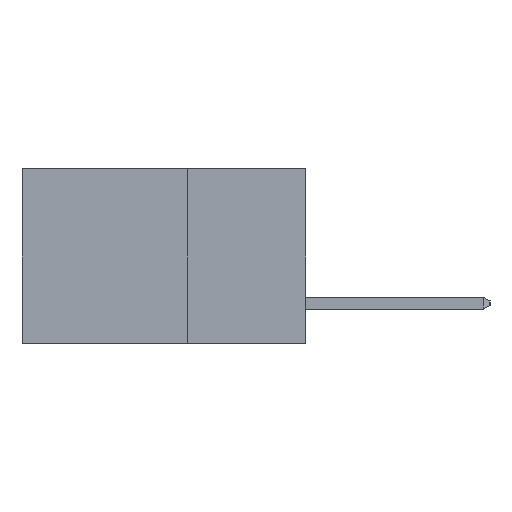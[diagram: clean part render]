
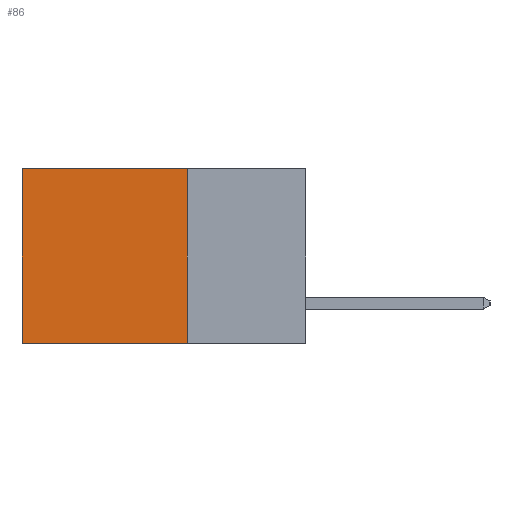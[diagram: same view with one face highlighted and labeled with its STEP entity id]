
A CAD part, left-side view. The second image highlights one B-rep face of the part: STEP entity #86.
In plain terms, the highlighted planar face has unit normal (-1, 0, 0).
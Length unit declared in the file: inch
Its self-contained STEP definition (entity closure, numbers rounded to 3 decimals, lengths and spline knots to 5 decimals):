
#24 = CARTESIAN_POINT ( 'NONE',  ( 0.2615, 0.25, -0.37 ) ) ;
#86 = ADVANCED_FACE ( 'NONE', ( #5015 ), #9644, .F. ) ;
#387 = CARTESIAN_POINT ( 'NONE',  ( 0.2615, 0.6, -0.37 ) ) ;
#1354 = DIRECTION ( 'NONE',  ( 0., 0., -1. ) ) ;
#1418 = AXIS2_PLACEMENT_3D ( 'NONE', #1578, #8172, #13003 ) ;
#1578 = CARTESIAN_POINT ( 'NONE',  ( 0.2615, 0.25, -0.37 ) ) ;
#2103 = EDGE_LOOP ( 'NONE', ( #4500, #5108, #12164, #8286 ) ) ;
#2274 = LINE ( 'NONE', #387, #12182 ) ;
#3090 = EDGE_CURVE ( 'NONE', #9852, #3947, #7965, .T. ) ;
#3339 = EDGE_CURVE ( 'NONE', #11125, #7864, #6919, .T. ) ;
#3477 = VECTOR ( 'NONE', #1354, 39.37008 ) ;
#3947 = VERTEX_POINT ( 'NONE', #9550 ) ;
#4035 = VECTOR ( 'NONE', #11109, 39.37008 ) ;
#4500 = ORIENTED_EDGE ( 'NONE', *, *, #14766, .T. ) ;
#4514 = CARTESIAN_POINT ( 'NONE',  ( 0.2615, 0.25, -0.37 ) ) ;
#5015 = FACE_OUTER_BOUND ( 'NONE', #2103, .T. ) ;
#5108 = ORIENTED_EDGE ( 'NONE', *, *, #3339, .F. ) ;
#5744 = DIRECTION ( 'NONE',  ( 0., 1., 0. ) ) ;
#6919 = LINE ( 'NONE', #10249, #9940 ) ;
#7864 = VERTEX_POINT ( 'NONE', #8886 ) ;
#7965 = LINE ( 'NONE', #10849, #4035 ) ;
#8172 = DIRECTION ( 'NONE',  ( 1., 0., 0. ) ) ;
#8286 = ORIENTED_EDGE ( 'NONE', *, *, #3090, .T. ) ;
#8290 = DIRECTION ( 'NONE',  ( 0., 0., -1. ) ) ;
#8485 = CARTESIAN_POINT ( 'NONE',  ( 0.2615, 0.25, 0. ) ) ;
#8886 = CARTESIAN_POINT ( 'NONE',  ( 0.2615, 0.6, -0.37 ) ) ;
#9550 = CARTESIAN_POINT ( 'NONE',  ( 0.2615, 0.6, 0. ) ) ;
#9644 = PLANE ( 'NONE',  #1418 ) ;
#9852 = VERTEX_POINT ( 'NONE', #8485 ) ;
#9940 = VECTOR ( 'NONE', #5744, 39.37008 ) ;
#10249 = CARTESIAN_POINT ( 'NONE',  ( 0.2615, 0.25, -0.37 ) ) ;
#10788 = LINE ( 'NONE', #24, #3477 ) ;
#10849 = CARTESIAN_POINT ( 'NONE',  ( 0.2615, 0.25, 0. ) ) ;
#11109 = DIRECTION ( 'NONE',  ( 0., 1., 0. ) ) ;
#11125 = VERTEX_POINT ( 'NONE', #4514 ) ;
#12164 = ORIENTED_EDGE ( 'NONE', *, *, #15510, .F. ) ;
#12182 = VECTOR ( 'NONE', #8290, 39.37008 ) ;
#13003 = DIRECTION ( 'NONE',  ( 0., 0., -1. ) ) ;
#14766 = EDGE_CURVE ( 'NONE', #3947, #7864, #2274, .T. ) ;
#15510 = EDGE_CURVE ( 'NONE', #9852, #11125, #10788, .T. ) ;
